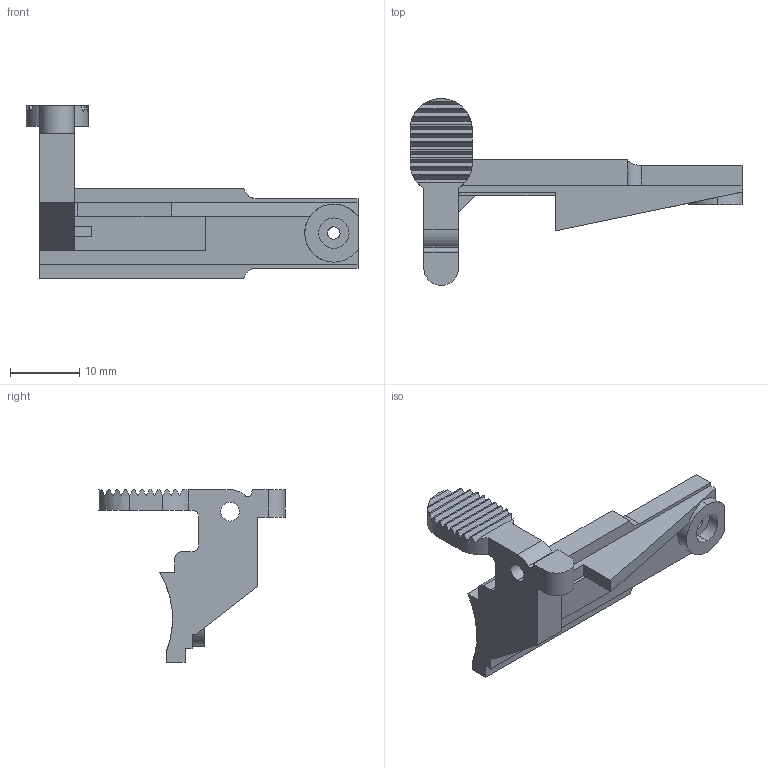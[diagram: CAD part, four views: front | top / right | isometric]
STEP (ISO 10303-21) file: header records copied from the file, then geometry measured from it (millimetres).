
FILE_DESCRIPTION (( 'STEP AP203' ), '1' );
FILE_NAME ('bolt_catch.STEP', '2021-12-29T04:07:58', ( '' ), ( '' ), 'SwSTEP 2.0', 'SolidWorks 2015', '' );
FILE_SCHEMA (( 'CONFIG_CONTROL_DESIGN' ));
Length unit declared in the file: millimetre
Products named in the file (1): bolt_catch
Bounding box: 48 x 27 x 25 mm (x, y, z)
Volume: 3095.6 mm3; surface area: 2818.6 mm2
Topology: 1 solids, 1 shells, 93 faces, 265 edges, 175 vertices
Faces by surface type: plane 70, cylinder 23
Entity records: 3136 total; most frequent: CARTESIAN_POINT 669, ORIENTED_EDGE 530, DIRECTION 473, EDGE_CURVE 265, VECTOR 179, LINE 179, VERTEX_POINT 175, AXIS2_PLACEMENT_3D 147
